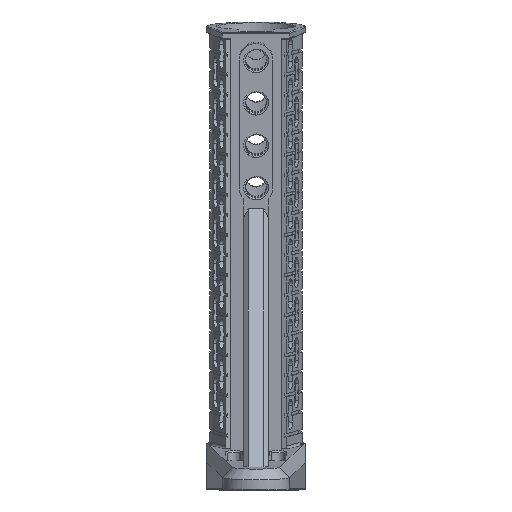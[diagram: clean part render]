
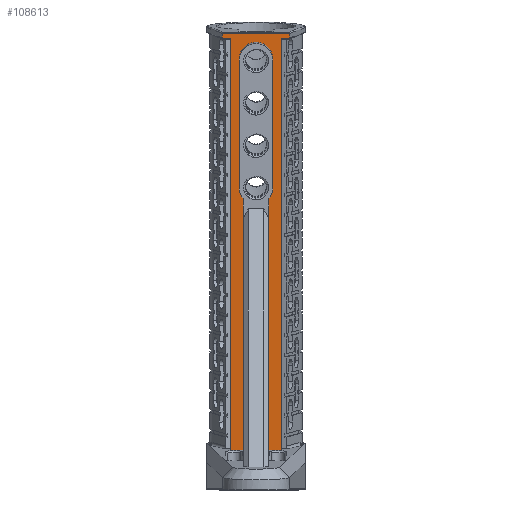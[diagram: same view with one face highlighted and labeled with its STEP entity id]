
A CAD part, left-side view. The second image highlights one B-rep face of the part: STEP entity #108613.
In plain terms, the highlighted planar face has unit normal (-0.996, 0, -0.087).
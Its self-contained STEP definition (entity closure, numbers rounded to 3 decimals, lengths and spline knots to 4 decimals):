
#1 = EDGE_CURVE ( 'NONE', #19655, #11546, #45817, .T. ) ;
#295 = CARTESIAN_POINT ( 'NONE',  ( -1.0606, -0.375, -0.1771 ) ) ;
#574 = VERTEX_POINT ( 'NONE', #50598 ) ;
#759 = DIRECTION ( 'NONE',  ( 0., 1., 0. ) ) ;
#1210 = VECTOR ( 'NONE', #33854, 39.3701 ) ;
#1700 = CARTESIAN_POINT ( 'NONE',  ( -0.5232, -0.375, -6.3196 ) ) ;
#7599 = ORIENTED_EDGE ( 'NONE', *, *, #77048, .T. ) ;
#8301 = VERTEX_POINT ( 'NONE', #45779 ) ;
#8627 = ORIENTED_EDGE ( 'NONE', *, *, #37814, .T. ) ;
#8632 = FACE_OUTER_BOUND ( 'NONE', #108732, .T. ) ;
#9136 = LINE ( 'NONE', #26437, #10490 ) ;
#9474 = EDGE_CURVE ( 'NONE', #76552, #31954, #87922, .T. ) ;
#9637 = LINE ( 'NONE', #16690, #1210 ) ;
#10332 = PLANE ( 'NONE',  #90936 ) ;
#10490 = VECTOR ( 'NONE', #71601, 39.3701 ) ;
#11240 = DIRECTION ( 'NONE',  ( -0.087, 0., 0.996 ) ) ;
#11546 = VERTEX_POINT ( 'NONE', #93629 ) ;
#11926 = CARTESIAN_POINT ( 'NONE',  ( -1.0592, 0.5, -0.193 ) ) ;
#14264 = EDGE_CURVE ( 'NONE', #57666, #19655, #41132, .T. ) ;
#14827 = LINE ( 'NONE', #77191, #60848 ) ;
#15464 = CARTESIAN_POINT ( 'NONE',  ( -0.5232, 0.375, -6.3196 ) ) ;
#15542 = DIRECTION ( 'NONE',  ( 0., -1., 0. ) ) ;
#16158 = ORIENTED_EDGE ( 'NONE', *, *, #65194, .T. ) ;
#16450 = VERTEX_POINT ( 'NONE', #79385 ) ;
#16690 = CARTESIAN_POINT ( 'NONE',  ( -0.8537, 0.1875, -2.5416 ) ) ;
#17647 = LINE ( 'NONE', #18803, #62266 ) ;
#17955 = DIRECTION ( 'NONE',  ( 0., -1., 0. ) ) ;
#18803 = CARTESIAN_POINT ( 'NONE',  ( -1.0665, -0.375, -0.1094 ) ) ;
#18830 = VECTOR ( 'NONE', #62279, 39.3701 ) ;
#19655 = VERTEX_POINT ( 'NONE', #77761 ) ;
#19746 = DIRECTION ( 'NONE',  ( 0., 1., 0. ) ) ;
#21411 = ORIENTED_EDGE ( 'NONE', *, *, #44576, .T. ) ;
#26437 = CARTESIAN_POINT ( 'NONE',  ( -1.0335, 0.25, -0.4869 ) ) ;
#26502 = DIRECTION ( 'NONE',  ( -0.087, 0., 0.996 ) ) ;
#26796 = CARTESIAN_POINT ( 'NONE',  ( -0.8674, 0.25, -2.3847 ) ) ;
#29334 = LINE ( 'NONE', #295, #89273 ) ;
#31143 = ORIENTED_EDGE ( 'NONE', *, *, #74378, .T. ) ;
#31707 = ORIENTED_EDGE ( 'NONE', *, *, #99931, .T. ) ;
#31954 = VERTEX_POINT ( 'NONE', #95104 ) ;
#33854 = DIRECTION ( 'NONE',  ( 0.087, 0., -0.996 ) ) ;
#35782 = DIRECTION ( 'NONE',  ( -0.996, 0., -0.087 ) ) ;
#35957 = LINE ( 'NONE', #90807, #94596 ) ;
#36125 = CARTESIAN_POINT ( 'NONE',  ( -1.0665, 0.5, -0.1094 ) ) ;
#37644 = DIRECTION ( 'NONE',  ( 0.087, 0., -0.996 ) ) ;
#37814 = EDGE_CURVE ( 'NONE', #81213, #81938, #86112, .T. ) ;
#38027 = DIRECTION ( 'NONE',  ( 0.087, 0., -0.996 ) ) ;
#38085 = AXIS2_PLACEMENT_3D ( 'NONE', #83445, #75224, #11240 ) ;
#39891 = VECTOR ( 'NONE', #37644, 39.3701 ) ;
#40008 = CARTESIAN_POINT ( 'NONE',  ( -0.5232, -0.375, -6.3196 ) ) ;
#40975 = CARTESIAN_POINT ( 'NONE',  ( -1.0606, -0.375, -0.1771 ) ) ;
#41132 = LINE ( 'NONE', #46762, #95671 ) ;
#42570 = ORIENTED_EDGE ( 'NONE', *, *, #113519, .F. ) ;
#42979 = VERTEX_POINT ( 'NONE', #113038 ) ;
#44576 = EDGE_CURVE ( 'NONE', #64018, #8301, #29334, .T. ) ;
#45558 = ORIENTED_EDGE ( 'NONE', *, *, #58902, .F. ) ;
#45779 = CARTESIAN_POINT ( 'NONE',  ( -1.0606, -0.5, -0.1771 ) ) ;
#45817 = CIRCLE ( 'NONE', #62410, 0.25 ) ;
#46242 = CARTESIAN_POINT ( 'NONE',  ( -0.4578, -0.375, -7.0668 ) ) ;
#46308 = DIRECTION ( 'NONE',  ( -0.087, 0., 0.996 ) ) ;
#46762 = CARTESIAN_POINT ( 'NONE',  ( -1.0335, -0.25, -0.4869 ) ) ;
#48661 = ORIENTED_EDGE ( 'NONE', *, *, #14264, .F. ) ;
#49641 = ORIENTED_EDGE ( 'NONE', *, *, #9474, .F. ) ;
#50418 = CARTESIAN_POINT ( 'NONE',  ( -1.0335, 0., -0.4869 ) ) ;
#50598 = CARTESIAN_POINT ( 'NONE',  ( -0.853, 0.1875, -2.5494 ) ) ;
#52198 = VERTEX_POINT ( 'NONE', #26796 ) ;
#54050 = LINE ( 'NONE', #1700, #86186 ) ;
#54166 = CIRCLE ( 'NONE', #54778, 0.25 ) ;
#54778 = AXIS2_PLACEMENT_3D ( 'NONE', #79915, #35782, #26502 ) ;
#55119 = CARTESIAN_POINT ( 'NONE',  ( -0.853, -0.1875, -2.5494 ) ) ;
#55610 = CARTESIAN_POINT ( 'NONE',  ( -0.8537, -0.1875, -2.5416 ) ) ;
#56315 = EDGE_CURVE ( 'NONE', #52198, #574, #54166, .T. ) ;
#56504 = DIRECTION ( 'NONE',  ( -0.087, 0., 0.996 ) ) ;
#57666 = VERTEX_POINT ( 'NONE', #64404 ) ;
#58070 = EDGE_CURVE ( 'NONE', #11546, #52198, #9136, .T. ) ;
#58902 = EDGE_CURVE ( 'NONE', #81213, #86810, #90013, .T. ) ;
#59280 = VECTOR ( 'NONE', #56504, 39.3701 ) ;
#59571 = VECTOR ( 'NONE', #15542, 39.3701 ) ;
#59593 = CARTESIAN_POINT ( 'NONE',  ( -0.5232, -0.375, -6.3196 ) ) ;
#60584 = CIRCLE ( 'NONE', #38085, 0.25 ) ;
#60848 = VECTOR ( 'NONE', #67786, 39.3701 ) ;
#62266 = VECTOR ( 'NONE', #759, 39.3701 ) ;
#62279 = DIRECTION ( 'NONE',  ( -0.087, 0., 0.996 ) ) ;
#62410 = AXIS2_PLACEMENT_3D ( 'NONE', #50418, #112913, #77767 ) ;
#64018 = VERTEX_POINT ( 'NONE', #40975 ) ;
#64404 = CARTESIAN_POINT ( 'NONE',  ( -0.8674, -0.25, -2.3847 ) ) ;
#64792 = VERTEX_POINT ( 'NONE', #55119 ) ;
#65015 = LINE ( 'NONE', #55610, #39891 ) ;
#65194 = EDGE_CURVE ( 'NONE', #64792, #31954, #65015, .T. ) ;
#67664 = LINE ( 'NONE', #74056, #59280 ) ;
#67786 = DIRECTION ( 'NONE',  ( -0.087, 0., 0.996 ) ) ;
#68970 = CARTESIAN_POINT ( 'NONE',  ( -1.0606, -0.375, -0.1771 ) ) ;
#70499 = ORIENTED_EDGE ( 'NONE', *, *, #56315, .F. ) ;
#71601 = DIRECTION ( 'NONE',  ( 0.087, 0., -0.996 ) ) ;
#72929 = DIRECTION ( 'NONE',  ( -0.087, 0., 0.996 ) ) ;
#73512 = DIRECTION ( 'NONE',  ( 0.996, 0., 0.087 ) ) ;
#74056 = CARTESIAN_POINT ( 'NONE',  ( -1.0592, -0.5, -0.193 ) ) ;
#74378 = EDGE_CURVE ( 'NONE', #16450, #86810, #17647, .T. ) ;
#75224 = DIRECTION ( 'NONE',  ( -0.996, 0., -0.087 ) ) ;
#76552 = VERTEX_POINT ( 'NONE', #59593 ) ;
#77048 = EDGE_CURVE ( 'NONE', #8301, #16450, #67664, .T. ) ;
#77191 = CARTESIAN_POINT ( 'NONE',  ( -0.4578, -0.375, -7.0668 ) ) ;
#77761 = CARTESIAN_POINT ( 'NONE',  ( -1.0335, -0.25, -0.4869 ) ) ;
#77767 = DIRECTION ( 'NONE',  ( -0.087, 0., 0.996 ) ) ;
#79385 = CARTESIAN_POINT ( 'NONE',  ( -1.0665, -0.5, -0.1094 ) ) ;
#79915 = CARTESIAN_POINT ( 'NONE',  ( -0.8674, 0., -2.3847 ) ) ;
#81213 = VERTEX_POINT ( 'NONE', #96146 ) ;
#81938 = VERTEX_POINT ( 'NONE', #92439 ) ;
#82362 = ORIENTED_EDGE ( 'NONE', *, *, #113987, .F. ) ;
#83445 = CARTESIAN_POINT ( 'NONE',  ( -0.8674, 0., -2.3847 ) ) ;
#83895 = VECTOR ( 'NONE', #102069, 39.3701 ) ;
#86112 = LINE ( 'NONE', #68970, #59571 ) ;
#86186 = VECTOR ( 'NONE', #19746, 39.3701 ) ;
#86459 = ORIENTED_EDGE ( 'NONE', *, *, #86735, .F. ) ;
#86735 = EDGE_CURVE ( 'NONE', #42979, #96233, #54050, .T. ) ;
#86810 = VERTEX_POINT ( 'NONE', #36125 ) ;
#87922 = LINE ( 'NONE', #40008, #83895 ) ;
#89273 = VECTOR ( 'NONE', #17955, 39.3701 ) ;
#90013 = LINE ( 'NONE', #11926, #18830 ) ;
#90807 = CARTESIAN_POINT ( 'NONE',  ( -0.4578, 0.375, -7.0668 ) ) ;
#90936 = AXIS2_PLACEMENT_3D ( 'NONE', #46242, #73512, #38027 ) ;
#92439 = CARTESIAN_POINT ( 'NONE',  ( -1.0606, 0.375, -0.1771 ) ) ;
#93629 = CARTESIAN_POINT ( 'NONE',  ( -1.0335, 0.25, -0.4869 ) ) ;
#94596 = VECTOR ( 'NONE', #46308, 39.3701 ) ;
#95104 = CARTESIAN_POINT ( 'NONE',  ( -0.5232, -0.1875, -6.3196 ) ) ;
#95671 = VECTOR ( 'NONE', #72929, 39.3701 ) ;
#96146 = CARTESIAN_POINT ( 'NONE',  ( -1.0606, 0.5, -0.1771 ) ) ;
#96233 = VERTEX_POINT ( 'NONE', #15464 ) ;
#99931 = EDGE_CURVE ( 'NONE', #76552, #64018, #14827, .T. ) ;
#102069 = DIRECTION ( 'NONE',  ( 0., 1., 0. ) ) ;
#102591 = ORIENTED_EDGE ( 'NONE', *, *, #58070, .F. ) ;
#105765 = ORIENTED_EDGE ( 'NONE', *, *, #113762, .F. ) ;
#107785 = ORIENTED_EDGE ( 'NONE', *, *, #1, .F. ) ;
#108613 = ADVANCED_FACE ( 'NONE', ( #8632 ), #10332, .F. ) ;
#108732 = EDGE_LOOP ( 'NONE', ( #31707, #21411, #7599, #31143, #45558, #8627, #42570, #86459, #82362, #70499, #102591, #107785, #48661, #105765, #16158, #49641 ) ) ;
#112913 = DIRECTION ( 'NONE',  ( -0.996, 0., -0.087 ) ) ;
#113038 = CARTESIAN_POINT ( 'NONE',  ( -0.5232, 0.1875, -6.3196 ) ) ;
#113519 = EDGE_CURVE ( 'NONE', #96233, #81938, #35957, .T. ) ;
#113762 = EDGE_CURVE ( 'NONE', #64792, #57666, #60584, .T. ) ;
#113987 = EDGE_CURVE ( 'NONE', #574, #42979, #9637, .T. ) ;
